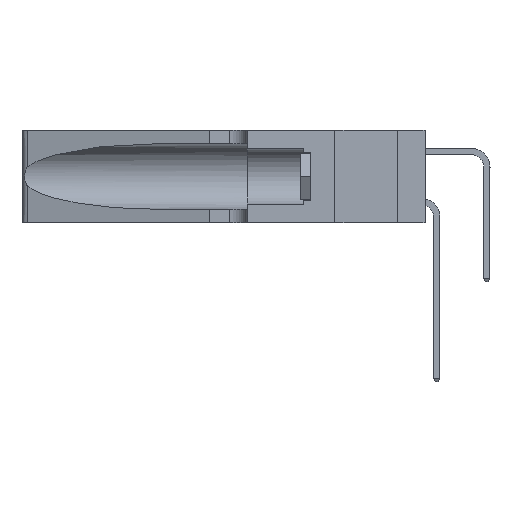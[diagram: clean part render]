
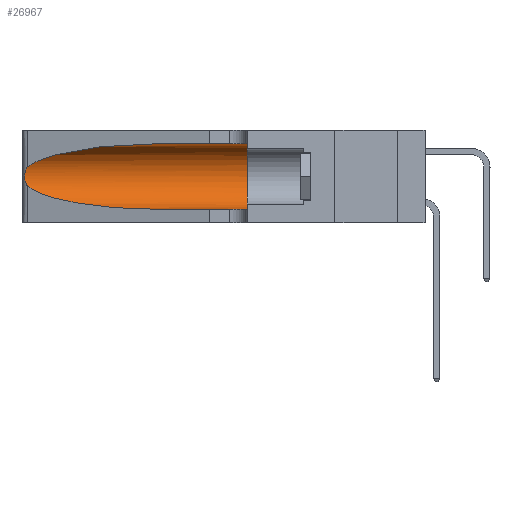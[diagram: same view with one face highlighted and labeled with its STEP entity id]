
A CAD part, left-side view. The second image highlights one B-rep face of the part: STEP entity #26967.
In plain terms, the highlighted cylindrical face has radius 3.308 mm (diameter 6.617 mm), a partial arc.
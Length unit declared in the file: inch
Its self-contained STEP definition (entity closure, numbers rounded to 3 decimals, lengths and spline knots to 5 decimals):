
#216 = CARTESIAN_POINT ( 'NONE',  ( 0.1305, 0.72297, 0.31525 ) ) ;
#550 = FACE_OUTER_BOUND ( 'NONE', #7846, .T. ) ;
#1106 = DIRECTION ( 'NONE',  ( 0., 1., 0. ) ) ;
#1730 = EDGE_CURVE ( 'NONE', #30155, #7294, #10665, .T. ) ;
#1846 = VERTEX_POINT ( 'NONE', #5865 ) ;
#2619 =( BOUNDED_CURVE ( )  B_SPLINE_CURVE ( 3, ( #14052, #26640, #34027, #41568 ),
 .UNSPECIFIED., .F., .T. ) 
 B_SPLINE_CURVE_WITH_KNOTS ( ( 4, 4 ),
 ( 3.44316, 4.71239 ),
 .UNSPECIFIED. ) 
 CURVE ( )  GEOMETRIC_REPRESENTATION_ITEM ( )  RATIONAL_B_SPLINE_CURVE ( ( 1., 0.87, 0.87, 1. ) ) 
 REPRESENTATION_ITEM ( '' )  );
#3532 = EDGE_CURVE ( 'NONE', #24966, #24454, #29467, .T. ) ;
#3806 = CARTESIAN_POINT ( 'NONE',  ( 0.1305, 0.35, 0.05475 ) ) ;
#4012 = CARTESIAN_POINT ( 'NONE',  ( 0.26017, 1.23833, 0.17102 ) ) ;
#4499 = ORIENTED_EDGE ( 'NONE', *, *, #12953, .F. ) ;
#5004 = AXIS2_PLACEMENT_3D ( 'NONE', #44226, #30936, #6492 ) ;
#5865 = CARTESIAN_POINT ( 'NONE',  ( 0.1305, 0.72297, 0.31525 ) ) ;
#6037 = CARTESIAN_POINT ( 'NONE',  ( 0.1305, 0.72297, 0.05475 ) ) ;
#6492 = DIRECTION ( 'NONE',  ( 0., 0., -1. ) ) ;
#7294 = VERTEX_POINT ( 'NONE', #18231 ) ;
#7371 = CARTESIAN_POINT ( 'NONE',  ( 0.25787, 1.23484, 0.2124 ) ) ;
#7639 = VECTOR ( 'NONE', #42904, 39.37008 ) ;
#7846 = EDGE_LOOP ( 'NONE', ( #23858, #35341, #18966, #25237, #27865, #4499 ) ) ;
#10665 = B_SPLINE_CURVE_WITH_KNOTS ( 'NONE', 3,
 ( #38529, #19255, #41488, #7371, #28069, #24267, #34805, #17061, #4012, #38635, #22233, #16341, #44521, #25949 ),
 .UNSPECIFIED., .F., .F.,
 ( 4, 2, 2, 2, 2, 2, 4 ),
 ( 0., 0.00027, 0.00053, 0.00107, 0.0016, 0.00187, 0.00214 ),
 .UNSPECIFIED. ) ;
#11081 = CARTESIAN_POINT ( 'NONE',  ( 0.1305, 0.35, 0.185 ) ) ;
#12236 = EDGE_CURVE ( 'NONE', #7294, #24966, #2619, .T. ) ;
#12953 = EDGE_CURVE ( 'NONE', #1846, #39874, #16329, .T. ) ;
#13550 = CARTESIAN_POINT ( 'NONE',  ( 0.25487, 1.22718, 0.22369 ) ) ;
#14052 = CARTESIAN_POINT ( 'NONE',  ( 0.25487, 1.22718, 0.14631 ) ) ;
#14111 = CYLINDRICAL_SURFACE ( 'NONE', #5004, 0.13025 ) ;
#16329 = LINE ( 'NONE', #39619, #7639 ) ;
#16341 = CARTESIAN_POINT ( 'NONE',  ( 0.25639, 1.23186, 0.15144 ) ) ;
#17061 = CARTESIAN_POINT ( 'NONE',  ( 0.26075, 1.23896, 0.178 ) ) ;
#18231 = CARTESIAN_POINT ( 'NONE',  ( 0.25487, 1.22718, 0.14631 ) ) ;
#18966 = ORIENTED_EDGE ( 'NONE', *, *, #12236, .T. ) ;
#19255 = CARTESIAN_POINT ( 'NONE',  ( 0.25555, 1.22994, 0.2215 ) ) ;
#22222 = CIRCLE ( 'NONE', #35954, 0.13025 ) ;
#22233 = CARTESIAN_POINT ( 'NONE',  ( 0.25789, 1.23486, 0.15765 ) ) ;
#23858 = ORIENTED_EDGE ( 'NONE', *, *, #43457, .T. ) ;
#24267 = CARTESIAN_POINT ( 'NONE',  ( 0.26018, 1.23835, 0.19895 ) ) ;
#24454 = VERTEX_POINT ( 'NONE', #3806 ) ;
#24966 = VERTEX_POINT ( 'NONE', #6037 ) ;
#25237 = ORIENTED_EDGE ( 'NONE', *, *, #3532, .T. ) ;
#25276 = DIRECTION ( 'NONE',  ( 0., 0., 1. ) ) ;
#25949 = CARTESIAN_POINT ( 'NONE',  ( 0.25487, 1.22718, 0.14631 ) ) ;
#26544 = EDGE_CURVE ( 'NONE', #39874, #24454, #22222, .T. ) ;
#26640 = CARTESIAN_POINT ( 'NONE',  ( 0.2373, 1.15595, 0.08982 ) ) ;
#26967 = ADVANCED_FACE ( 'NONE', ( #550 ), #14111, .F. ) ;
#27865 = ORIENTED_EDGE ( 'NONE', *, *, #26544, .F. ) ;
#28069 = CARTESIAN_POINT ( 'NONE',  ( 0.25854, 1.2359, 0.20912 ) ) ;
#28390 = VECTOR ( 'NONE', #37529, 39.37008 ) ;
#28979 = CARTESIAN_POINT ( 'NONE',  ( 0.25487, 1.22718, 0.22369 ) ) ;
#29467 = LINE ( 'NONE', #36202, #28390 ) ;
#30155 = VERTEX_POINT ( 'NONE', #28979 ) ;
#30727 = CARTESIAN_POINT ( 'NONE',  ( 0.18966, 0.96281, 0.31525 ) ) ;
#30936 = DIRECTION ( 'NONE',  ( 0., -1., 0. ) ) ;
#33396 = CARTESIAN_POINT ( 'NONE',  ( 0.1305, 0.35, 0.31525 ) ) ;
#34027 = CARTESIAN_POINT ( 'NONE',  ( 0.18966, 0.96281, 0.05475 ) ) ;
#34805 = CARTESIAN_POINT ( 'NONE',  ( 0.26075, 1.23896, 0.19203 ) ) ;
#35341 = ORIENTED_EDGE ( 'NONE', *, *, #1730, .T. ) ;
#35954 = AXIS2_PLACEMENT_3D ( 'NONE', #11081, #1106, #25276 ) ;
#36202 = CARTESIAN_POINT ( 'NONE',  ( 0.1305, 1.61858, 0.05475 ) ) ;
#37529 = DIRECTION ( 'NONE',  ( 0., -1., 0. ) ) ;
#38529 = CARTESIAN_POINT ( 'NONE',  ( 0.25487, 1.22718, 0.22369 ) ) ;
#38635 = CARTESIAN_POINT ( 'NONE',  ( 0.25856, 1.23593, 0.16098 ) ) ;
#39619 = CARTESIAN_POINT ( 'NONE',  ( 0.1305, 1.61858, 0.31525 ) ) ;
#39874 = VERTEX_POINT ( 'NONE', #33396 ) ;
#41123 = CARTESIAN_POINT ( 'NONE',  ( 0.2373, 1.15595, 0.28018 ) ) ;
#41488 = CARTESIAN_POINT ( 'NONE',  ( 0.25639, 1.23184, 0.21858 ) ) ;
#41568 = CARTESIAN_POINT ( 'NONE',  ( 0.1305, 0.72297, 0.05475 ) ) ;
#42904 = DIRECTION ( 'NONE',  ( 0., -1., 0. ) ) ;
#43332 =( BOUNDED_CURVE ( )  B_SPLINE_CURVE ( 3, ( #216, #30727, #41123, #13550 ),
 .UNSPECIFIED., .F., .F. ) 
 B_SPLINE_CURVE_WITH_KNOTS ( ( 4, 4 ),
 ( 1.5708, 2.84003 ),
 .UNSPECIFIED. ) 
 CURVE ( )  GEOMETRIC_REPRESENTATION_ITEM ( )  RATIONAL_B_SPLINE_CURVE ( ( 1., 0.87, 0.87, 1. ) ) 
 REPRESENTATION_ITEM ( '' )  );
#43457 = EDGE_CURVE ( 'NONE', #1846, #30155, #43332, .T. ) ;
#44226 = CARTESIAN_POINT ( 'NONE',  ( 0.1305, 1.61858, 0.185 ) ) ;
#44521 = CARTESIAN_POINT ( 'NONE',  ( 0.25555, 1.22993, 0.14849 ) ) ;
